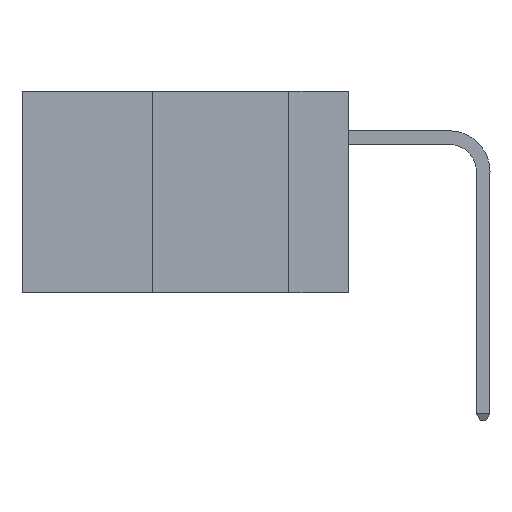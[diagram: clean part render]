
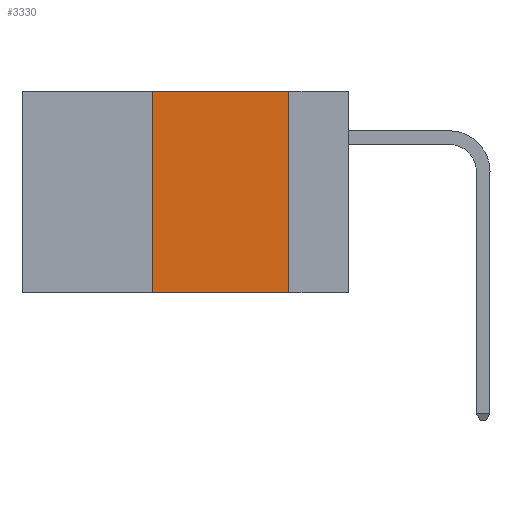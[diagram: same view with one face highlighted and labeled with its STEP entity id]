
A CAD part, left-side view. The second image highlights one B-rep face of the part: STEP entity #3330.
In plain terms, the highlighted planar face has unit normal (-1, 0, 0).
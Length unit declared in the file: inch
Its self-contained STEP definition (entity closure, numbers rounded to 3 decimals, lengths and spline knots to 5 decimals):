
#5 = DIRECTION ( 'NONE',  ( 0., 0., 1. ) ) ;
#222 = VERTEX_POINT ( 'NONE', #3121 ) ;
#286 = VECTOR ( 'NONE', #509, 39.37008 ) ;
#509 = DIRECTION ( 'NONE',  ( 0., -1., 0. ) ) ;
#527 = VERTEX_POINT ( 'NONE', #6149 ) ;
#754 = CARTESIAN_POINT ( 'NONE',  ( 0., 0.36, -0.37 ) ) ;
#779 = VECTOR ( 'NONE', #3245, 39.37008 ) ;
#994 = VERTEX_POINT ( 'NONE', #6912 ) ;
#1259 = FACE_OUTER_BOUND ( 'NONE', #1299, .T. ) ;
#1299 = EDGE_LOOP ( 'NONE', ( #6630, #6888, #7083, #7389 ) ) ;
#1702 = PLANE ( 'NONE',  #10134 ) ;
#1856 = VERTEX_POINT ( 'NONE', #754 ) ;
#2753 = DIRECTION ( 'NONE',  ( 1., 0., 0. ) ) ;
#3121 = CARTESIAN_POINT ( 'NONE',  ( 0., 0.11, 0. ) ) ;
#3146 = CARTESIAN_POINT ( 'NONE',  ( 0., 0.11, 0. ) ) ;
#3245 = DIRECTION ( 'NONE',  ( 0., -1., 0. ) ) ;
#3330 = ADVANCED_FACE ( 'NONE', ( #1259 ), #1702, .F. ) ;
#4551 = LINE ( 'NONE', #8651, #286 ) ;
#6011 = LINE ( 'NONE', #10291, #779 ) ;
#6149 = CARTESIAN_POINT ( 'NONE',  ( 0., 0.11, -0.37 ) ) ;
#6190 = EDGE_CURVE ( 'NONE', #994, #222, #4551, .T. ) ;
#6630 = ORIENTED_EDGE ( 'NONE', *, *, #8169, .F. ) ;
#6771 = CARTESIAN_POINT ( 'NONE',  ( 0., 0.36, 0. ) ) ;
#6888 = ORIENTED_EDGE ( 'NONE', *, *, #6190, .F. ) ;
#6912 = CARTESIAN_POINT ( 'NONE',  ( 0., 0.36, 0. ) ) ;
#7083 = ORIENTED_EDGE ( 'NONE', *, *, #8197, .F. ) ;
#7221 = CARTESIAN_POINT ( 'NONE',  ( 0., 0.6, 0. ) ) ;
#7389 = ORIENTED_EDGE ( 'NONE', *, *, #8246, .T. ) ;
#7933 = VECTOR ( 'NONE', #5, 39.37008 ) ;
#8169 = EDGE_CURVE ( 'NONE', #222, #527, #9898, .T. ) ;
#8197 = EDGE_CURVE ( 'NONE', #1856, #994, #9487, .T. ) ;
#8246 = EDGE_CURVE ( 'NONE', #1856, #527, #6011, .T. ) ;
#8651 = CARTESIAN_POINT ( 'NONE',  ( 0., 0.6, 0. ) ) ;
#8699 = DIRECTION ( 'NONE',  ( 0., 0., -1. ) ) ;
#9487 = LINE ( 'NONE', #6771, #7933 ) ;
#9530 = VECTOR ( 'NONE', #9709, 39.37008 ) ;
#9709 = DIRECTION ( 'NONE',  ( 0., 0., -1. ) ) ;
#9898 = LINE ( 'NONE', #3146, #9530 ) ;
#10134 = AXIS2_PLACEMENT_3D ( 'NONE', #7221, #2753, #8699 ) ;
#10291 = CARTESIAN_POINT ( 'NONE',  ( 0., 0.6, -0.37 ) ) ;
